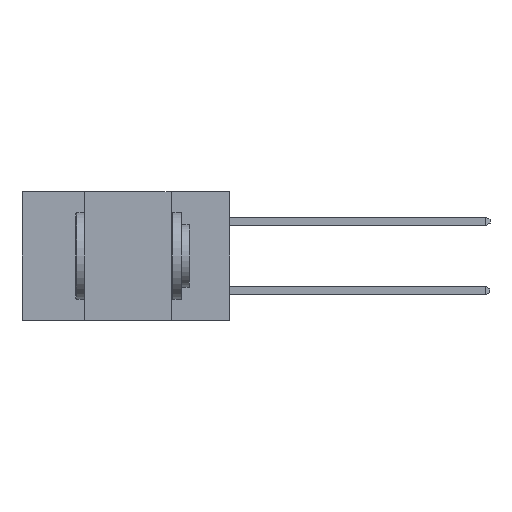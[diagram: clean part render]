
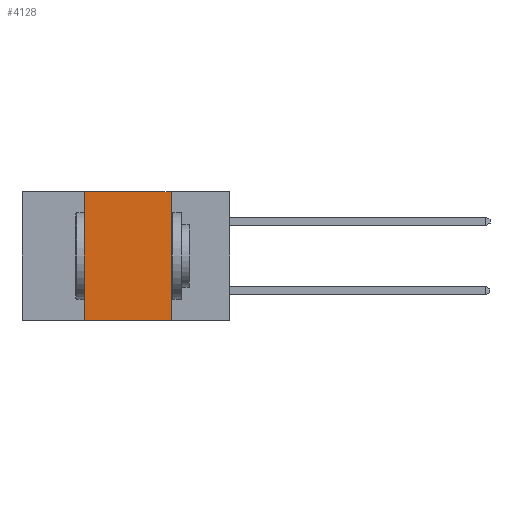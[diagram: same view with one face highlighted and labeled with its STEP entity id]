
A CAD part, left-side view. The second image highlights one B-rep face of the part: STEP entity #4128.
In plain terms, the highlighted planar face has unit normal (-1, 0, 0).
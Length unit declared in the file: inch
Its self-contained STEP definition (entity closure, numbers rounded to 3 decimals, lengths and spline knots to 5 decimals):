
#367 = DIRECTION ( 'NONE',  ( 0., -1., 0. ) ) ;
#463 = LINE ( 'NONE', #6608, #7766 ) ;
#1358 = VERTEX_POINT ( 'NONE', #1874 ) ;
#1740 = CARTESIAN_POINT ( 'NONE',  ( 0., 0.6, 0. ) ) ;
#1751 = AXIS2_PLACEMENT_3D ( 'NONE', #1740, #8430, #8401 ) ;
#1874 = CARTESIAN_POINT ( 'NONE',  ( 0., 0.17, 0. ) ) ;
#1898 = VECTOR ( 'NONE', #5925, 39.37008 ) ;
#2994 = CARTESIAN_POINT ( 'NONE',  ( 0., 0.42, 0. ) ) ;
#3094 = VERTEX_POINT ( 'NONE', #4825 ) ;
#3391 = CARTESIAN_POINT ( 'NONE',  ( 0., 0.17, 0. ) ) ;
#3630 = EDGE_CURVE ( 'NONE', #3094, #1358, #7682, .T. ) ;
#4128 = ADVANCED_FACE ( 'NONE', ( #12462 ), #12543, .F. ) ;
#4409 = VERTEX_POINT ( 'NONE', #5602 ) ;
#4825 = CARTESIAN_POINT ( 'NONE',  ( 0., 0.42, 0. ) ) ;
#5066 = VECTOR ( 'NONE', #367, 39.37008 ) ;
#5268 = ORIENTED_EDGE ( 'NONE', *, *, #3630, .F. ) ;
#5334 = ORIENTED_EDGE ( 'NONE', *, *, #10249, .F. ) ;
#5602 = CARTESIAN_POINT ( 'NONE',  ( 0., 0.17, -0.37 ) ) ;
#5645 = EDGE_CURVE ( 'NONE', #1358, #4409, #12257, .T. ) ;
#5925 = DIRECTION ( 'NONE',  ( 0., 0., -1. ) ) ;
#6085 = EDGE_CURVE ( 'NONE', #12356, #4409, #463, .T. ) ;
#6608 = CARTESIAN_POINT ( 'NONE',  ( 0., 0.6, -0.37 ) ) ;
#7450 = VECTOR ( 'NONE', #12655, 39.37008 ) ;
#7682 = LINE ( 'NONE', #9438, #5066 ) ;
#7766 = VECTOR ( 'NONE', #11235, 39.37008 ) ;
#8401 = DIRECTION ( 'NONE',  ( 0., 0., -1. ) ) ;
#8430 = DIRECTION ( 'NONE',  ( 1., 0., 0. ) ) ;
#9438 = CARTESIAN_POINT ( 'NONE',  ( 0., 0.6, 0. ) ) ;
#9778 = EDGE_LOOP ( 'NONE', ( #11074, #5268, #5334, #12118 ) ) ;
#10249 = EDGE_CURVE ( 'NONE', #12356, #3094, #12529, .T. ) ;
#11074 = ORIENTED_EDGE ( 'NONE', *, *, #5645, .F. ) ;
#11235 = DIRECTION ( 'NONE',  ( 0., -1., 0. ) ) ;
#11287 = CARTESIAN_POINT ( 'NONE',  ( 0., 0.42, -0.37 ) ) ;
#12118 = ORIENTED_EDGE ( 'NONE', *, *, #6085, .T. ) ;
#12257 = LINE ( 'NONE', #3391, #1898 ) ;
#12356 = VERTEX_POINT ( 'NONE', #11287 ) ;
#12462 = FACE_OUTER_BOUND ( 'NONE', #9778, .T. ) ;
#12529 = LINE ( 'NONE', #2994, #7450 ) ;
#12543 = PLANE ( 'NONE',  #1751 ) ;
#12655 = DIRECTION ( 'NONE',  ( 0., 0., 1. ) ) ;
